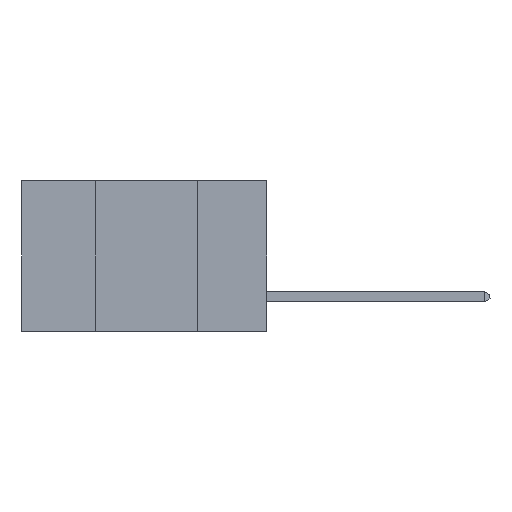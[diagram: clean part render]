
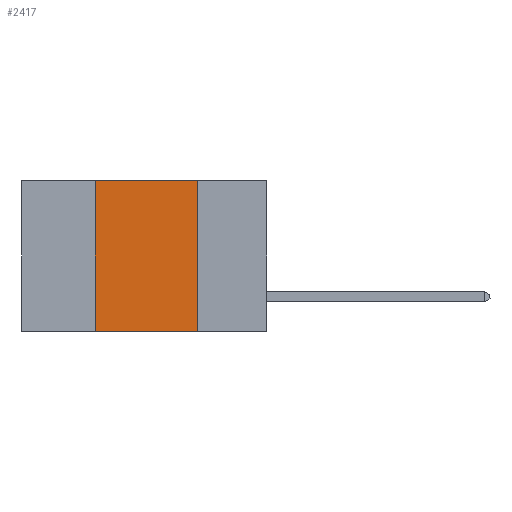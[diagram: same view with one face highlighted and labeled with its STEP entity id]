
A CAD part, left-side view. The second image highlights one B-rep face of the part: STEP entity #2417.
In plain terms, the highlighted planar face has unit normal (-1, 0, 0).
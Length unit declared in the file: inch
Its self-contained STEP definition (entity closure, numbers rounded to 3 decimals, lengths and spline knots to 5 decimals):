
#1749 = PLANE ( 'NONE',  #13090 ) ;
#2151 = EDGE_LOOP ( 'NONE', ( #6584, #6895, #5651, #12016 ) ) ;
#2202 = LINE ( 'NONE', #7505, #10263 ) ;
#2231 = DIRECTION ( 'NONE',  ( 0., 0., 1. ) ) ;
#2417 = ADVANCED_FACE ( 'NONE', ( #4904 ), #1749, .F. ) ;
#2429 = CARTESIAN_POINT ( 'NONE',  ( 0., 0.42, -0.37 ) ) ;
#2670 = EDGE_CURVE ( 'NONE', #13484, #5624, #2202, .T. ) ;
#2868 = DIRECTION ( 'NONE',  ( 1., 0., 0. ) ) ;
#2900 = LINE ( 'NONE', #8568, #8233 ) ;
#3254 = LINE ( 'NONE', #13118, #8244 ) ;
#4904 = FACE_OUTER_BOUND ( 'NONE', #2151, .T. ) ;
#5577 = CARTESIAN_POINT ( 'NONE',  ( 0., 0.17, 0. ) ) ;
#5624 = VERTEX_POINT ( 'NONE', #8318 ) ;
#5651 = ORIENTED_EDGE ( 'NONE', *, *, #11358, .F. ) ;
#5939 = EDGE_CURVE ( 'NONE', #9672, #5624, #9585, .T. ) ;
#6063 = DIRECTION ( 'NONE',  ( 0., -1., 0. ) ) ;
#6584 = ORIENTED_EDGE ( 'NONE', *, *, #5939, .F. ) ;
#6681 = DIRECTION ( 'NONE',  ( 0., 0., -1. ) ) ;
#6895 = ORIENTED_EDGE ( 'NONE', *, *, #8425, .F. ) ;
#7505 = CARTESIAN_POINT ( 'NONE',  ( 0., 0.6, -0.37 ) ) ;
#8183 = CARTESIAN_POINT ( 'NONE',  ( 0., 0.6, 0. ) ) ;
#8233 = VECTOR ( 'NONE', #2231, 39.37008 ) ;
#8244 = VECTOR ( 'NONE', #6063, 39.37008 ) ;
#8318 = CARTESIAN_POINT ( 'NONE',  ( 0., 0.17, -0.37 ) ) ;
#8425 = EDGE_CURVE ( 'NONE', #11782, #9672, #3254, .T. ) ;
#8540 = DIRECTION ( 'NONE',  ( 0., -1., 0. ) ) ;
#8568 = CARTESIAN_POINT ( 'NONE',  ( 0., 0.42, 0. ) ) ;
#9211 = CARTESIAN_POINT ( 'NONE',  ( 0., 0.17, 0. ) ) ;
#9585 = LINE ( 'NONE', #5577, #9900 ) ;
#9672 = VERTEX_POINT ( 'NONE', #9211 ) ;
#9900 = VECTOR ( 'NONE', #6681, 39.37008 ) ;
#10207 = DIRECTION ( 'NONE',  ( 0., 0., -1. ) ) ;
#10263 = VECTOR ( 'NONE', #8540, 39.37008 ) ;
#11358 = EDGE_CURVE ( 'NONE', #13484, #11782, #2900, .T. ) ;
#11782 = VERTEX_POINT ( 'NONE', #12289 ) ;
#12016 = ORIENTED_EDGE ( 'NONE', *, *, #2670, .T. ) ;
#12289 = CARTESIAN_POINT ( 'NONE',  ( 0., 0.42, 0. ) ) ;
#13090 = AXIS2_PLACEMENT_3D ( 'NONE', #8183, #2868, #10207 ) ;
#13118 = CARTESIAN_POINT ( 'NONE',  ( 0., 0.6, 0. ) ) ;
#13484 = VERTEX_POINT ( 'NONE', #2429 ) ;
